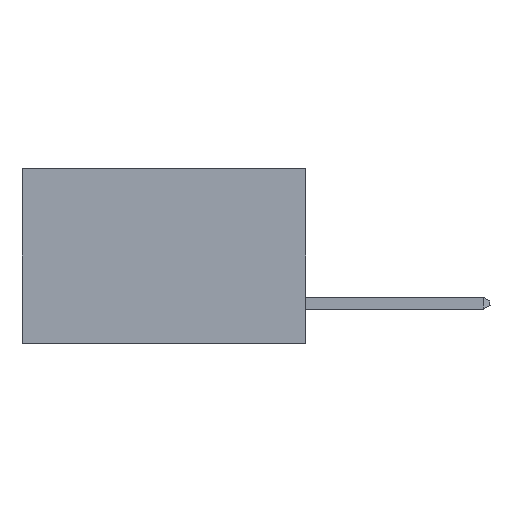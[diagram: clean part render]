
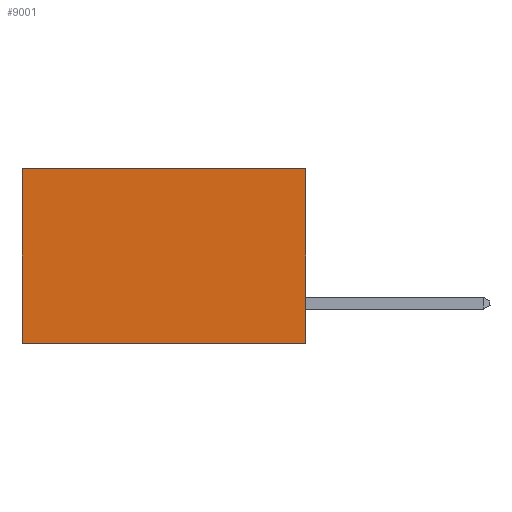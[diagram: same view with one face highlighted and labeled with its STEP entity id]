
A CAD part, left-side view. The second image highlights one B-rep face of the part: STEP entity #9001.
In plain terms, the highlighted planar face has unit normal (-1, 0, 0).
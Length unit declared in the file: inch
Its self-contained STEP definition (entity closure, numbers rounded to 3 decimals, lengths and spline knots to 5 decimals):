
#1251 = CARTESIAN_POINT ( 'NONE',  ( 0.298, 0.6, 0. ) ) ;
#2823 = ORIENTED_EDGE ( 'NONE', *, *, #18605, .T. ) ;
#3816 = ORIENTED_EDGE ( 'NONE', *, *, #11696, .F. ) ;
#4786 = DIRECTION ( 'NONE',  ( 0., 0., -1. ) ) ;
#5297 = LINE ( 'NONE', #13093, #6533 ) ;
#5685 = LINE ( 'NONE', #19813, #10743 ) ;
#6533 = VECTOR ( 'NONE', #4786, 39.37008 ) ;
#6790 = ORIENTED_EDGE ( 'NONE', *, *, #19957, .T. ) ;
#7060 = DIRECTION ( 'NONE',  ( 0., 0., -1. ) ) ;
#7123 = LINE ( 'NONE', #20568, #19184 ) ;
#7125 = VERTEX_POINT ( 'NONE', #17448 ) ;
#7407 = VERTEX_POINT ( 'NONE', #8627 ) ;
#8312 = EDGE_CURVE ( 'NONE', #7125, #12696, #5685, .T. ) ;
#8389 = EDGE_LOOP ( 'NONE', ( #6790, #11795, #3816, #2823 ) ) ;
#8627 = CARTESIAN_POINT ( 'NONE',  ( 0.298, 0., 0. ) ) ;
#9001 = ADVANCED_FACE ( 'NONE', ( #18940 ), #17082, .F. ) ;
#10455 = DIRECTION ( 'NONE',  ( 0., 1., 0. ) ) ;
#10743 = VECTOR ( 'NONE', #16636, 39.37008 ) ;
#11118 = DIRECTION ( 'NONE',  ( 0., 0., -1. ) ) ;
#11696 = EDGE_CURVE ( 'NONE', #7407, #7125, #5297, .T. ) ;
#11795 = ORIENTED_EDGE ( 'NONE', *, *, #8312, .F. ) ;
#11887 = AXIS2_PLACEMENT_3D ( 'NONE', #13618, #18746, #7060 ) ;
#12696 = VERTEX_POINT ( 'NONE', #20750 ) ;
#13093 = CARTESIAN_POINT ( 'NONE',  ( 0.298, 0., 0. ) ) ;
#13618 = CARTESIAN_POINT ( 'NONE',  ( 0.298, 0., 0. ) ) ;
#14769 = VERTEX_POINT ( 'NONE', #1251 ) ;
#15014 = CARTESIAN_POINT ( 'NONE',  ( 0.298, 0., 0. ) ) ;
#16636 = DIRECTION ( 'NONE',  ( 0., 1., 0. ) ) ;
#17082 = PLANE ( 'NONE',  #11887 ) ;
#17448 = CARTESIAN_POINT ( 'NONE',  ( 0.298, 0., -0.37 ) ) ;
#18511 = LINE ( 'NONE', #15014, #21052 ) ;
#18605 = EDGE_CURVE ( 'NONE', #7407, #14769, #18511, .T. ) ;
#18746 = DIRECTION ( 'NONE',  ( 1., 0., 0. ) ) ;
#18940 = FACE_OUTER_BOUND ( 'NONE', #8389, .T. ) ;
#19184 = VECTOR ( 'NONE', #11118, 39.37008 ) ;
#19813 = CARTESIAN_POINT ( 'NONE',  ( 0.298, 0., -0.37 ) ) ;
#19957 = EDGE_CURVE ( 'NONE', #14769, #12696, #7123, .T. ) ;
#20568 = CARTESIAN_POINT ( 'NONE',  ( 0.298, 0.6, 0. ) ) ;
#20750 = CARTESIAN_POINT ( 'NONE',  ( 0.298, 0.6, -0.37 ) ) ;
#21052 = VECTOR ( 'NONE', #10455, 39.37008 ) ;
